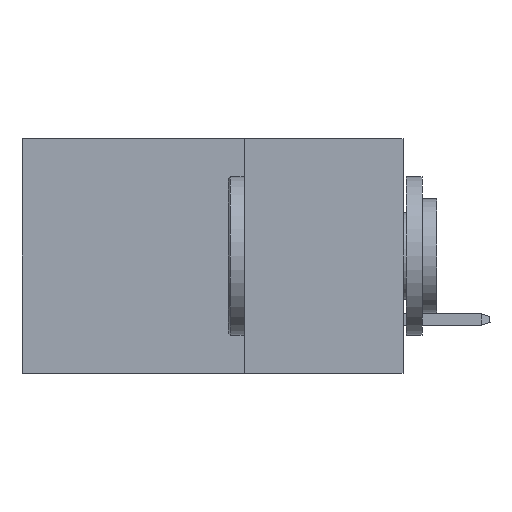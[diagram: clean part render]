
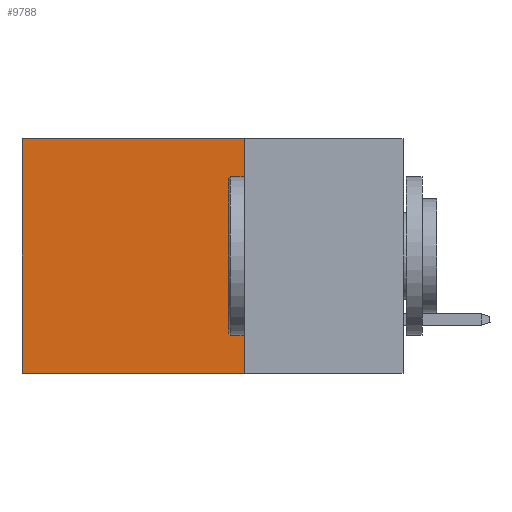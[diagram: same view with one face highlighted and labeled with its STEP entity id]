
A CAD part, left-side view. The second image highlights one B-rep face of the part: STEP entity #9788.
In plain terms, the highlighted planar face has unit normal (-1, 0, 0).
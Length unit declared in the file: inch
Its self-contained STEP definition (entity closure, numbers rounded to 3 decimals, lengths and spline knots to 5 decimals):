
#656 = DIRECTION ( 'NONE',  ( 0., 1., 0. ) ) ;
#2061 = CARTESIAN_POINT ( 'NONE',  ( 0.2875, 0.6, -0.37 ) ) ;
#4385 = EDGE_CURVE ( 'NONE', #31925, #36854, #30744, .T. ) ;
#4875 = VECTOR ( 'NONE', #656, 39.37008 ) ;
#5271 = DIRECTION ( 'NONE',  ( 0., 0., -1. ) ) ;
#5291 = ORIENTED_EDGE ( 'NONE', *, *, #38216, .F. ) ;
#5946 = VERTEX_POINT ( 'NONE', #11635 ) ;
#7947 = VECTOR ( 'NONE', #16272, 39.37008 ) ;
#9366 = ORIENTED_EDGE ( 'NONE', *, *, #4385, .T. ) ;
#9788 = ADVANCED_FACE ( 'NONE', ( #33298 ), #33987, .F. ) ;
#11100 = DIRECTION ( 'NONE',  ( 0., 1., 0. ) ) ;
#11538 = LINE ( 'NONE', #21898, #19157 ) ;
#11635 = CARTESIAN_POINT ( 'NONE',  ( 0.2875, 0.25, -0.37 ) ) ;
#11883 = CARTESIAN_POINT ( 'NONE',  ( 0.2875, 0.25, 0. ) ) ;
#12183 = CARTESIAN_POINT ( 'NONE',  ( 0.2875, 0.25, -0.37 ) ) ;
#13327 = CARTESIAN_POINT ( 'NONE',  ( 0.2875, 0.6, 0. ) ) ;
#16272 = DIRECTION ( 'NONE',  ( 0., 0., -1. ) ) ;
#19043 = AXIS2_PLACEMENT_3D ( 'NONE', #11883, #26241, #5271 ) ;
#19157 = VECTOR ( 'NONE', #11100, 39.37008 ) ;
#19624 = VERTEX_POINT ( 'NONE', #25320 ) ;
#21898 = CARTESIAN_POINT ( 'NONE',  ( 0.2875, 0.25, 0. ) ) ;
#25320 = CARTESIAN_POINT ( 'NONE',  ( 0.2875, 0.25, 0. ) ) ;
#26241 = DIRECTION ( 'NONE',  ( 1., 0., 0. ) ) ;
#28636 = ORIENTED_EDGE ( 'NONE', *, *, #42747, .T. ) ;
#30641 = LINE ( 'NONE', #45216, #7947 ) ;
#30744 = LINE ( 'NONE', #13327, #39519 ) ;
#31925 = VERTEX_POINT ( 'NONE', #34990 ) ;
#33298 = FACE_OUTER_BOUND ( 'NONE', #37076, .T. ) ;
#33610 = ORIENTED_EDGE ( 'NONE', *, *, #37237, .F. ) ;
#33987 = PLANE ( 'NONE',  #19043 ) ;
#34513 = DIRECTION ( 'NONE',  ( 0., 0., -1. ) ) ;
#34990 = CARTESIAN_POINT ( 'NONE',  ( 0.2875, 0.6, 0. ) ) ;
#36854 = VERTEX_POINT ( 'NONE', #2061 ) ;
#36925 = LINE ( 'NONE', #12183, #4875 ) ;
#37076 = EDGE_LOOP ( 'NONE', ( #9366, #33610, #5291, #28636 ) ) ;
#37237 = EDGE_CURVE ( 'NONE', #5946, #36854, #36925, .T. ) ;
#38216 = EDGE_CURVE ( 'NONE', #19624, #5946, #30641, .T. ) ;
#39519 = VECTOR ( 'NONE', #34513, 39.37008 ) ;
#42747 = EDGE_CURVE ( 'NONE', #19624, #31925, #11538, .T. ) ;
#45216 = CARTESIAN_POINT ( 'NONE',  ( 0.2875, 0.25, 0. ) ) ;
